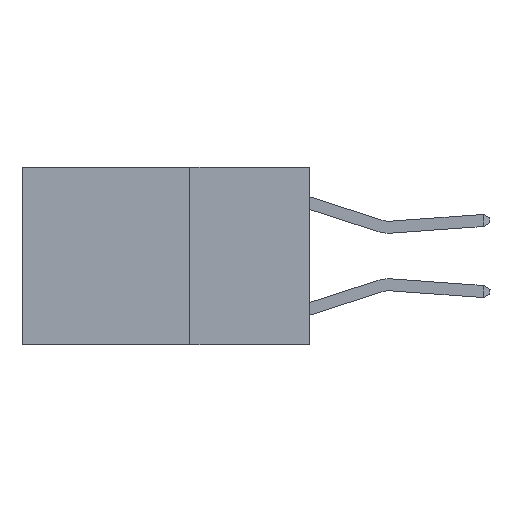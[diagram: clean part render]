
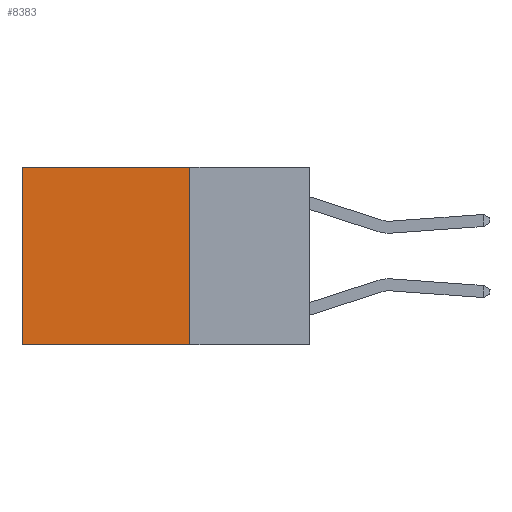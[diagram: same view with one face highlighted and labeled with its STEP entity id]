
A CAD part, left-side view. The second image highlights one B-rep face of the part: STEP entity #8383.
In plain terms, the highlighted planar face has unit normal (-1, 0, 0).
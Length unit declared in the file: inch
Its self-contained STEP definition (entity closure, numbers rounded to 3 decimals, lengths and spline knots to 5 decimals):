
#315 = CARTESIAN_POINT ( 'NONE',  ( 0.2625, 0.6, -0.37 ) ) ;
#356 = ORIENTED_EDGE ( 'NONE', *, *, #2913, .F. ) ;
#1128 = VERTEX_POINT ( 'NONE', #3935 ) ;
#1284 = DIRECTION ( 'NONE',  ( 0., 0., -1. ) ) ;
#1637 = CARTESIAN_POINT ( 'NONE',  ( 0.2625, 0.25, 0. ) ) ;
#2298 = LINE ( 'NONE', #20292, #19281 ) ;
#2690 = LINE ( 'NONE', #5252, #23988 ) ;
#2913 = EDGE_CURVE ( 'NONE', #14062, #13599, #14373, .T. ) ;
#3021 = EDGE_CURVE ( 'NONE', #14062, #1128, #22984, .T. ) ;
#3935 = CARTESIAN_POINT ( 'NONE',  ( 0.2625, 0.6, 0. ) ) ;
#5252 = CARTESIAN_POINT ( 'NONE',  ( 0.2625, 0.6, 0. ) ) ;
#6658 = EDGE_LOOP ( 'NONE', ( #19805, #26728, #356, #11060 ) ) ;
#6914 = CARTESIAN_POINT ( 'NONE',  ( 0.2625, 0.25, -0.37 ) ) ;
#8383 = ADVANCED_FACE ( 'NONE', ( #21122 ), #11955, .F. ) ;
#8786 = VERTEX_POINT ( 'NONE', #315 ) ;
#10413 = CARTESIAN_POINT ( 'NONE',  ( 0.2625, 0.25, 0. ) ) ;
#11060 = ORIENTED_EDGE ( 'NONE', *, *, #3021, .T. ) ;
#11955 = PLANE ( 'NONE',  #25692 ) ;
#13599 = VERTEX_POINT ( 'NONE', #6914 ) ;
#14062 = VERTEX_POINT ( 'NONE', #10413 ) ;
#14073 = DIRECTION ( 'NONE',  ( 0., 0., -1. ) ) ;
#14098 = DIRECTION ( 'NONE',  ( 1., 0., 0. ) ) ;
#14373 = LINE ( 'NONE', #20457, #19996 ) ;
#18677 = DIRECTION ( 'NONE',  ( 0., 1., 0. ) ) ;
#19281 = VECTOR ( 'NONE', #26460, 39.37008 ) ;
#19805 = ORIENTED_EDGE ( 'NONE', *, *, #23059, .T. ) ;
#19996 = VECTOR ( 'NONE', #14073, 39.37008 ) ;
#20292 = CARTESIAN_POINT ( 'NONE',  ( 0.2625, 0.25, -0.37 ) ) ;
#20457 = CARTESIAN_POINT ( 'NONE',  ( 0.2625, 0.25, 0. ) ) ;
#21122 = FACE_OUTER_BOUND ( 'NONE', #6658, .T. ) ;
#22242 = DIRECTION ( 'NONE',  ( 0., 0., -1. ) ) ;
#22319 = VECTOR ( 'NONE', #18677, 39.37008 ) ;
#22984 = LINE ( 'NONE', #1637, #22319 ) ;
#23059 = EDGE_CURVE ( 'NONE', #1128, #8786, #2690, .T. ) ;
#23988 = VECTOR ( 'NONE', #22242, 39.37008 ) ;
#24141 = EDGE_CURVE ( 'NONE', #13599, #8786, #2298, .T. ) ;
#25692 = AXIS2_PLACEMENT_3D ( 'NONE', #26766, #14098, #1284 ) ;
#26460 = DIRECTION ( 'NONE',  ( 0., 1., 0. ) ) ;
#26728 = ORIENTED_EDGE ( 'NONE', *, *, #24141, .F. ) ;
#26766 = CARTESIAN_POINT ( 'NONE',  ( 0.2625, 0.25, 0. ) ) ;
